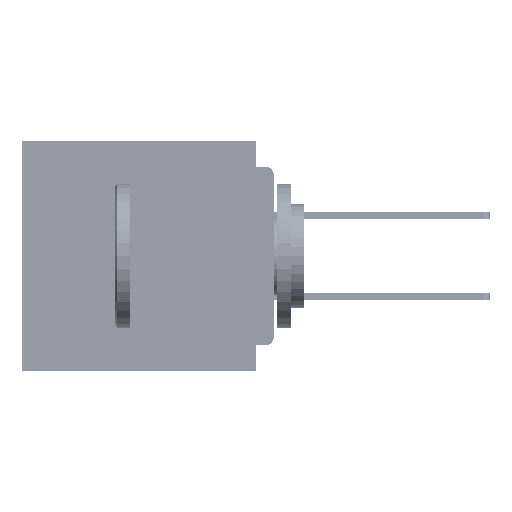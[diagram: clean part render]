
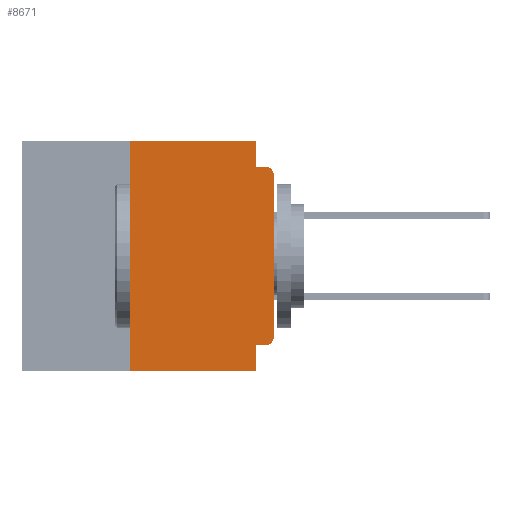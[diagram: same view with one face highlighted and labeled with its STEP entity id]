
A CAD part, left-side view. The second image highlights one B-rep face of the part: STEP entity #8671.
In plain terms, the highlighted planar face has unit normal (-1, 0, 0).
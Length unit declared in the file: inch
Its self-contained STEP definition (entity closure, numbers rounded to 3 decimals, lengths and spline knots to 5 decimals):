
#820 = CARTESIAN_POINT ( 'NONE',  ( 0., 0.25, -0.4 ) ) ;
#1321 = FACE_OUTER_BOUND ( 'NONE', #23856, .T. ) ;
#1748 = VERTEX_POINT ( 'NONE', #820 ) ;
#2309 = CARTESIAN_POINT ( 'NONE',  ( 0., 0.015, -0.34 ) ) ;
#2925 = AXIS2_PLACEMENT_3D ( 'NONE', #16561, #55064, #22118 ) ;
#3265 = CARTESIAN_POINT ( 'NONE',  ( 0., 0.437, 0. ) ) ;
#3451 = CARTESIAN_POINT ( 'NONE',  ( 0., 0., -0.045 ) ) ;
#3761 = EDGE_CURVE ( 'NONE', #1748, #69082, #63031, .T. ) ;
#4058 = VECTOR ( 'NONE', #70658, 39.37008 ) ;
#4536 = ORIENTED_EDGE ( 'NONE', *, *, #11019, .F. ) ;
#6729 = VERTEX_POINT ( 'NONE', #29196 ) ;
#7913 = DIRECTION ( 'NONE',  ( 0., 0., -1. ) ) ;
#8671 = ADVANCED_FACE ( 'NONE', ( #1321 ), #41749, .F. ) ;
#8846 = DIRECTION ( 'NONE',  ( 1., 0., 0. ) ) ;
#9438 = CARTESIAN_POINT ( 'NONE',  ( 0., 0.031, 0. ) ) ;
#10556 = AXIS2_PLACEMENT_3D ( 'NONE', #2309, #41054, #7913 ) ;
#11019 = EDGE_CURVE ( 'NONE', #20606, #31144, #27027, .T. ) ;
#12532 = EDGE_CURVE ( 'NONE', #56716, #6729, #41750, .T. ) ;
#15766 = EDGE_CURVE ( 'NONE', #43433, #70721, #44804, .T. ) ;
#16561 = CARTESIAN_POINT ( 'NONE',  ( 0., 0.015, -0.06 ) ) ;
#17439 = VECTOR ( 'NONE', #69337, 39.37008 ) ;
#19669 = CARTESIAN_POINT ( 'NONE',  ( 0., 0.015, -0.355 ) ) ;
#20277 = DIRECTION ( 'NONE',  ( 0., 1., 0. ) ) ;
#20606 = VERTEX_POINT ( 'NONE', #41188 ) ;
#22118 = DIRECTION ( 'NONE',  ( 0., 0., -1. ) ) ;
#22126 = ORIENTED_EDGE ( 'NONE', *, *, #70937, .F. ) ;
#22134 = CIRCLE ( 'NONE', #10556, 0.015 ) ;
#23162 = ORIENTED_EDGE ( 'NONE', *, *, #24197, .T. ) ;
#23463 = VECTOR ( 'NONE', #20277, 39.37008 ) ;
#23856 = EDGE_LOOP ( 'NONE', ( #69518, #39095, #49032, #4536, #42055, #54893, #54918, #38600, #22126, #23162 ) ) ;
#24153 = AXIS2_PLACEMENT_3D ( 'NONE', #3265, #8846, #47498 ) ;
#24197 = EDGE_CURVE ( 'NONE', #64110, #43433, #22134, .T. ) ;
#27027 = LINE ( 'NONE', #9438, #51120 ) ;
#27061 = VECTOR ( 'NONE', #37782, 39.37008 ) ;
#28854 = CARTESIAN_POINT ( 'NONE',  ( 0., 0.25, -0.4 ) ) ;
#29196 = CARTESIAN_POINT ( 'NONE',  ( 0., 0.031, -0.4 ) ) ;
#31144 = VERTEX_POINT ( 'NONE', #66908 ) ;
#32754 = CARTESIAN_POINT ( 'NONE',  ( 0., 0.437, 0. ) ) ;
#33857 = VECTOR ( 'NONE', #45282, 39.37008 ) ;
#35329 = DIRECTION ( 'NONE',  ( 0., 0., 1. ) ) ;
#37782 = DIRECTION ( 'NONE',  ( 0., 0., -1. ) ) ;
#38091 = LINE ( 'NONE', #47748, #23463 ) ;
#38364 = EDGE_CURVE ( 'NONE', #69082, #20606, #70820, .T. ) ;
#38600 = ORIENTED_EDGE ( 'NONE', *, *, #12532, .F. ) ;
#39095 = ORIENTED_EDGE ( 'NONE', *, *, #63719, .T. ) ;
#40326 = CARTESIAN_POINT ( 'NONE',  ( 0., 0., -0.06 ) ) ;
#41054 = DIRECTION ( 'NONE',  ( -1., 0., 0. ) ) ;
#41188 = CARTESIAN_POINT ( 'NONE',  ( 0., 0.031, 0. ) ) ;
#41749 = PLANE ( 'NONE',  #24153 ) ;
#41750 = LINE ( 'NONE', #65033, #27061 ) ;
#41859 = VECTOR ( 'NONE', #70783, 39.37008 ) ;
#42055 = ORIENTED_EDGE ( 'NONE', *, *, #38364, .F. ) ;
#42577 = DIRECTION ( 'NONE',  ( 0., 0., -1. ) ) ;
#43433 = VERTEX_POINT ( 'NONE', #66270 ) ;
#44623 = VERTEX_POINT ( 'NONE', #50572 ) ;
#44804 = LINE ( 'NONE', #51705, #59308 ) ;
#45282 = DIRECTION ( 'NONE',  ( 0., 0., 1. ) ) ;
#46479 = LINE ( 'NONE', #65221, #4058 ) ;
#46712 = EDGE_CURVE ( 'NONE', #31144, #44623, #46752, .T. ) ;
#46752 = LINE ( 'NONE', #3451, #17439 ) ;
#47498 = DIRECTION ( 'NONE',  ( 0., 0., -1. ) ) ;
#47748 = CARTESIAN_POINT ( 'NONE',  ( 0., 0., -0.355 ) ) ;
#49032 = ORIENTED_EDGE ( 'NONE', *, *, #46712, .F. ) ;
#50572 = CARTESIAN_POINT ( 'NONE',  ( 0., 0.015, -0.045 ) ) ;
#51120 = VECTOR ( 'NONE', #42577, 39.37008 ) ;
#51705 = CARTESIAN_POINT ( 'NONE',  ( 0., 0., 0. ) ) ;
#51943 = CIRCLE ( 'NONE', #2925, 0.015 ) ;
#52116 = CARTESIAN_POINT ( 'NONE',  ( 0., 0.25, 0. ) ) ;
#54893 = ORIENTED_EDGE ( 'NONE', *, *, #3761, .F. ) ;
#54918 = ORIENTED_EDGE ( 'NONE', *, *, #67089, .T. ) ;
#55064 = DIRECTION ( 'NONE',  ( -1., 0., 0. ) ) ;
#56716 = VERTEX_POINT ( 'NONE', #64822 ) ;
#59308 = VECTOR ( 'NONE', #35329, 39.37008 ) ;
#63031 = LINE ( 'NONE', #28854, #33857 ) ;
#63719 = EDGE_CURVE ( 'NONE', #70721, #44623, #51943, .T. ) ;
#64110 = VERTEX_POINT ( 'NONE', #19669 ) ;
#64822 = CARTESIAN_POINT ( 'NONE',  ( 0., 0.031, -0.355 ) ) ;
#65033 = CARTESIAN_POINT ( 'NONE',  ( 0., 0.031, -0.4 ) ) ;
#65221 = CARTESIAN_POINT ( 'NONE',  ( 0., 0.437, -0.4 ) ) ;
#66270 = CARTESIAN_POINT ( 'NONE',  ( 0., 0., -0.34 ) ) ;
#66908 = CARTESIAN_POINT ( 'NONE',  ( 0., 0.031, -0.045 ) ) ;
#67089 = EDGE_CURVE ( 'NONE', #1748, #6729, #46479, .T. ) ;
#69082 = VERTEX_POINT ( 'NONE', #52116 ) ;
#69337 = DIRECTION ( 'NONE',  ( 0., -1., 0. ) ) ;
#69518 = ORIENTED_EDGE ( 'NONE', *, *, #15766, .T. ) ;
#70658 = DIRECTION ( 'NONE',  ( 0., -1., 0. ) ) ;
#70721 = VERTEX_POINT ( 'NONE', #40326 ) ;
#70783 = DIRECTION ( 'NONE',  ( 0., -1., 0. ) ) ;
#70820 = LINE ( 'NONE', #32754, #41859 ) ;
#70937 = EDGE_CURVE ( 'NONE', #64110, #56716, #38091, .T. ) ;
